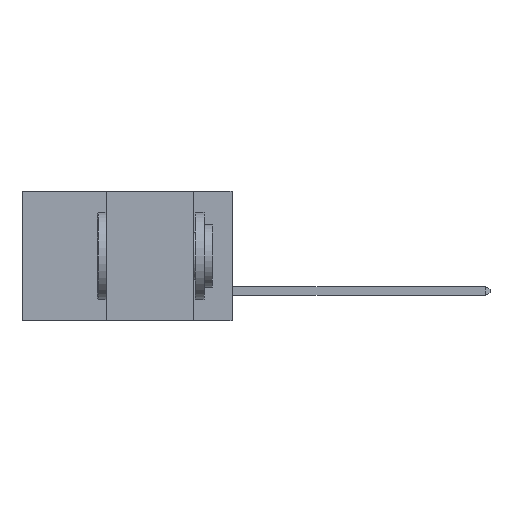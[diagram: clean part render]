
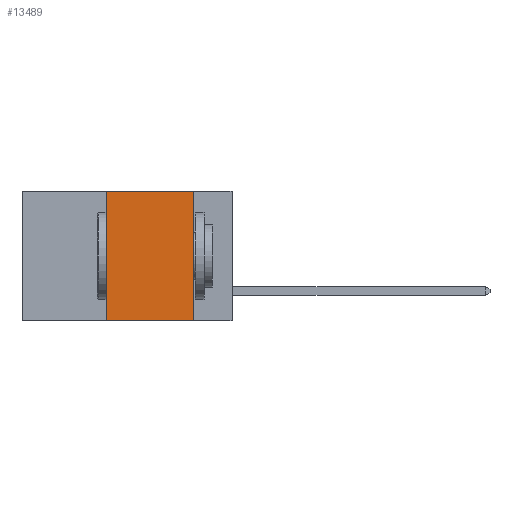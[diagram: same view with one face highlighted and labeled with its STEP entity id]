
A CAD part, left-side view. The second image highlights one B-rep face of the part: STEP entity #13489.
In plain terms, the highlighted planar face has unit normal (-1, 0, 0).
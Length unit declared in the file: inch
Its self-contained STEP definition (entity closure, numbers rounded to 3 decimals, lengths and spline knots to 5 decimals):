
#978 = EDGE_LOOP ( 'NONE', ( #2812, #13016, #28975, #5739 ) ) ;
#1107 = EDGE_CURVE ( 'NONE', #27615, #26411, #11472, .T. ) ;
#1645 = DIRECTION ( 'NONE',  ( 0., -1., 0. ) ) ;
#2422 = EDGE_CURVE ( 'NONE', #23071, #26411, #33444, .T. ) ;
#2812 = ORIENTED_EDGE ( 'NONE', *, *, #1107, .F. ) ;
#4144 = LINE ( 'NONE', #32518, #35398 ) ;
#4172 = CARTESIAN_POINT ( 'NONE',  ( 0., 0.6, -0.37 ) ) ;
#5739 = ORIENTED_EDGE ( 'NONE', *, *, #2422, .T. ) ;
#8013 = EDGE_CURVE ( 'NONE', #16188, #27615, #4144, .T. ) ;
#8023 = PLANE ( 'NONE',  #13788 ) ;
#11151 = DIRECTION ( 'NONE',  ( 0., 0., -1. ) ) ;
#11472 = LINE ( 'NONE', #32950, #25535 ) ;
#13016 = ORIENTED_EDGE ( 'NONE', *, *, #8013, .F. ) ;
#13489 = ADVANCED_FACE ( 'NONE', ( #20513 ), #8023, .F. ) ;
#13788 = AXIS2_PLACEMENT_3D ( 'NONE', #35053, #29169, #11151 ) ;
#15187 = CARTESIAN_POINT ( 'NONE',  ( 0., 0.36, -0.37 ) ) ;
#15559 = EDGE_CURVE ( 'NONE', #23071, #16188, #37325, .T. ) ;
#15683 = CARTESIAN_POINT ( 'NONE',  ( 0., 0.11, 0. ) ) ;
#16188 = VERTEX_POINT ( 'NONE', #22626 ) ;
#19641 = DIRECTION ( 'NONE',  ( 0., 0., 1. ) ) ;
#20325 = VECTOR ( 'NONE', #19641, 39.37008 ) ;
#20513 = FACE_OUTER_BOUND ( 'NONE', #978, .T. ) ;
#22626 = CARTESIAN_POINT ( 'NONE',  ( 0., 0.36, 0. ) ) ;
#23071 = VERTEX_POINT ( 'NONE', #15187 ) ;
#25434 = VECTOR ( 'NONE', #37370, 39.37008 ) ;
#25535 = VECTOR ( 'NONE', #33081, 39.37008 ) ;
#26411 = VERTEX_POINT ( 'NONE', #31141 ) ;
#27615 = VERTEX_POINT ( 'NONE', #15683 ) ;
#28975 = ORIENTED_EDGE ( 'NONE', *, *, #15559, .F. ) ;
#29169 = DIRECTION ( 'NONE',  ( 1., 0., 0. ) ) ;
#31141 = CARTESIAN_POINT ( 'NONE',  ( 0., 0.11, -0.37 ) ) ;
#31667 = CARTESIAN_POINT ( 'NONE',  ( 0., 0.36, 0. ) ) ;
#32518 = CARTESIAN_POINT ( 'NONE',  ( 0., 0.6, 0. ) ) ;
#32950 = CARTESIAN_POINT ( 'NONE',  ( 0., 0.11, 0. ) ) ;
#33081 = DIRECTION ( 'NONE',  ( 0., 0., -1. ) ) ;
#33444 = LINE ( 'NONE', #4172, #25434 ) ;
#35053 = CARTESIAN_POINT ( 'NONE',  ( 0., 0.6, 0. ) ) ;
#35398 = VECTOR ( 'NONE', #1645, 39.37008 ) ;
#37325 = LINE ( 'NONE', #31667, #20325 ) ;
#37370 = DIRECTION ( 'NONE',  ( 0., -1., 0. ) ) ;
